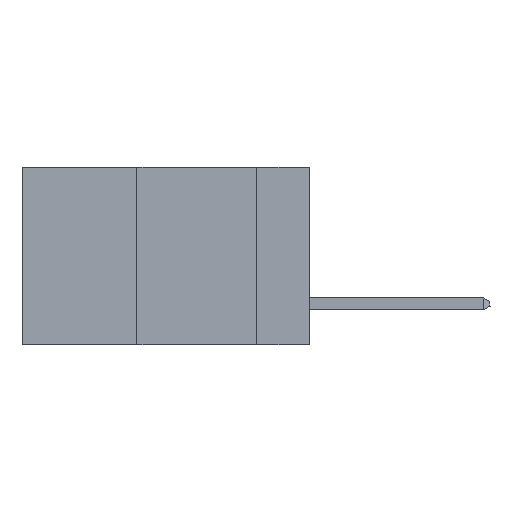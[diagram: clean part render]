
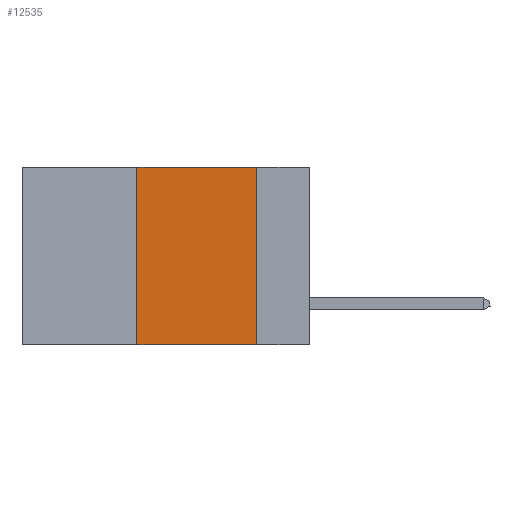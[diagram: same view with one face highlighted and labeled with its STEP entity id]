
A CAD part, left-side view. The second image highlights one B-rep face of the part: STEP entity #12535.
In plain terms, the highlighted planar face has unit normal (-1, 0, 0).
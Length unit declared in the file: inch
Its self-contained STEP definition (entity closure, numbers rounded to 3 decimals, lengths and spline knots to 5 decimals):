
#344 = CARTESIAN_POINT ( 'NONE',  ( 0., 0.6, 0. ) ) ;
#372 = VECTOR ( 'NONE', #3470, 39.37008 ) ;
#1886 = CARTESIAN_POINT ( 'NONE',  ( 0., 0.11, 0. ) ) ;
#2922 = VERTEX_POINT ( 'NONE', #10324 ) ;
#3470 = DIRECTION ( 'NONE',  ( 0., -1., 0. ) ) ;
#4359 = DIRECTION ( 'NONE',  ( 0., 0., -1. ) ) ;
#4575 = ORIENTED_EDGE ( 'NONE', *, *, #29460, .F. ) ;
#5387 = VECTOR ( 'NONE', #23425, 39.37008 ) ;
#5403 = ORIENTED_EDGE ( 'NONE', *, *, #15321, .F. ) ;
#6183 = VERTEX_POINT ( 'NONE', #25253 ) ;
#6440 = FACE_OUTER_BOUND ( 'NONE', #18217, .T. ) ;
#7965 = DIRECTION ( 'NONE',  ( 1., 0., 0. ) ) ;
#10324 = CARTESIAN_POINT ( 'NONE',  ( 0., 0.11, -0.37 ) ) ;
#10508 = EDGE_CURVE ( 'NONE', #11793, #15365, #21552, .T. ) ;
#10844 = LINE ( 'NONE', #1886, #12395 ) ;
#11143 = LINE ( 'NONE', #13575, #372 ) ;
#11793 = VERTEX_POINT ( 'NONE', #25151 ) ;
#12395 = VECTOR ( 'NONE', #4359, 39.37008 ) ;
#12535 = ADVANCED_FACE ( 'NONE', ( #6440 ), #22652, .F. ) ;
#12888 = DIRECTION ( 'NONE',  ( 0., 0., 1. ) ) ;
#13495 = ORIENTED_EDGE ( 'NONE', *, *, #10508, .F. ) ;
#13575 = CARTESIAN_POINT ( 'NONE',  ( 0., 0.6, 0. ) ) ;
#15321 = EDGE_CURVE ( 'NONE', #6183, #2922, #10844, .T. ) ;
#15365 = VERTEX_POINT ( 'NONE', #28993 ) ;
#18217 = EDGE_LOOP ( 'NONE', ( #5403, #4575, #13495, #24360 ) ) ;
#20783 = VECTOR ( 'NONE', #12888, 39.37008 ) ;
#21093 = CARTESIAN_POINT ( 'NONE',  ( 0., 0.6, -0.37 ) ) ;
#21552 = LINE ( 'NONE', #27526, #20783 ) ;
#22652 = PLANE ( 'NONE',  #24184 ) ;
#22863 = EDGE_CURVE ( 'NONE', #11793, #2922, #26478, .T. ) ;
#23425 = DIRECTION ( 'NONE',  ( 0., -1., 0. ) ) ;
#24184 = AXIS2_PLACEMENT_3D ( 'NONE', #344, #7965, #24699 ) ;
#24360 = ORIENTED_EDGE ( 'NONE', *, *, #22863, .T. ) ;
#24699 = DIRECTION ( 'NONE',  ( 0., 0., -1. ) ) ;
#25151 = CARTESIAN_POINT ( 'NONE',  ( 0., 0.36, -0.37 ) ) ;
#25253 = CARTESIAN_POINT ( 'NONE',  ( 0., 0.11, 0. ) ) ;
#26478 = LINE ( 'NONE', #21093, #5387 ) ;
#27526 = CARTESIAN_POINT ( 'NONE',  ( 0., 0.36, 0. ) ) ;
#28993 = CARTESIAN_POINT ( 'NONE',  ( 0., 0.36, 0. ) ) ;
#29460 = EDGE_CURVE ( 'NONE', #15365, #6183, #11143, .T. ) ;
